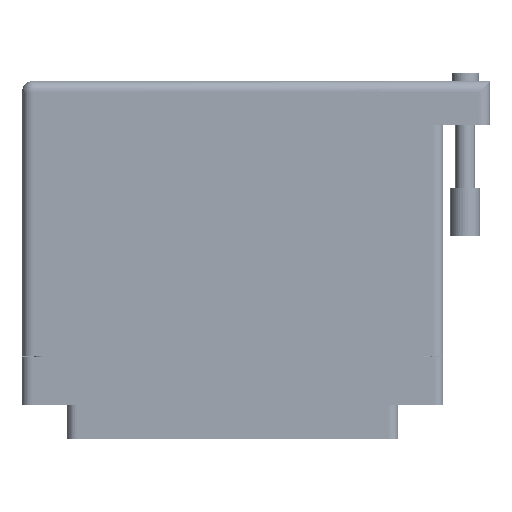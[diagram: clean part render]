
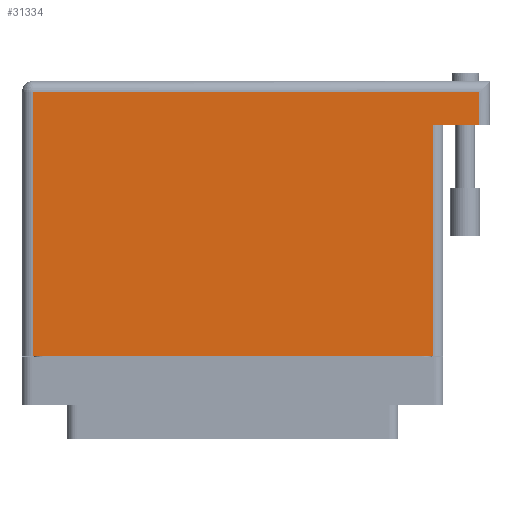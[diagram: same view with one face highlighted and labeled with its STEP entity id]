
A CAD part, front view. The second image highlights one B-rep face of the part: STEP entity #31334.
In plain terms, the highlighted face is planar.
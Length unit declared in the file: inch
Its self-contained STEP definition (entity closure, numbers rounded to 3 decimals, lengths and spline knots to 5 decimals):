
#239 = CARTESIAN_POINT ( 'NONE',  ( -1.289, -0.1, 0.617 ) ) ;
#4967 = ORIENTED_EDGE ( 'NONE', *, *, #35825, .T. ) ;
#5981 = VERTEX_POINT ( 'NONE', #13484 ) ;
#6640 = DIRECTION ( 'NONE',  ( 1., 0., 0. ) ) ;
#6830 = AXIS2_PLACEMENT_3D ( 'NONE', #13305, #51186, #57053 ) ;
#6877 = CARTESIAN_POINT ( 'NONE',  ( -1.359, -0.1, 0.617 ) ) ;
#6927 = ORIENTED_EDGE ( 'NONE', *, *, #57910, .F. ) ;
#8064 = EDGE_CURVE ( 'NONE', #47133, #68225, #53258, .T. ) ;
#10103 = FACE_OUTER_BOUND ( 'NONE', #64344, .T. ) ;
#10275 = ORIENTED_EDGE ( 'NONE', *, *, #18310, .T. ) ;
#11267 = VECTOR ( 'NONE', #66884, 39.37008 ) ;
#12974 = LINE ( 'NONE', #51051, #11267 ) ;
#13305 = CARTESIAN_POINT ( 'NONE',  ( -1.359, 1.675, 0.617 ) ) ;
#13484 = CARTESIAN_POINT ( 'NONE',  ( 1.589, 1.395, 0.617 ) ) ;
#13561 = VECTOR ( 'NONE', #64209, 39.37008 ) ;
#15276 = CARTESIAN_POINT ( 'NONE',  ( 1.289, 1.395, 0.617 ) ) ;
#16328 = ORIENTED_EDGE ( 'NONE', *, *, #60985, .T. ) ;
#17291 = LINE ( 'NONE', #48616, #28340 ) ;
#17690 = LINE ( 'NONE', #68873, #23637 ) ;
#17777 = LINE ( 'NONE', #26431, #13561 ) ;
#18310 = EDGE_CURVE ( 'NONE', #67453, #47133, #17777, .T. ) ;
#22267 = ORIENTED_EDGE ( 'NONE', *, *, #8064, .T. ) ;
#22354 = VECTOR ( 'NONE', #6640, 39.37008 ) ;
#23018 = CARTESIAN_POINT ( 'NONE',  ( -1.289, -0.1, 0.617 ) ) ;
#23637 = VECTOR ( 'NONE', #46229, 39.37008 ) ;
#26431 = CARTESIAN_POINT ( 'NONE',  ( -1.359, 1.605, 0.617 ) ) ;
#27829 = VERTEX_POINT ( 'NONE', #15276 ) ;
#28340 = VECTOR ( 'NONE', #59426, 39.37008 ) ;
#31334 = ADVANCED_FACE ( 'NONE', ( #10103 ), #67724, .F. ) ;
#33004 = ORIENTED_EDGE ( 'NONE', *, *, #51006, .T. ) ;
#34826 = CARTESIAN_POINT ( 'NONE',  ( 1.589, 1.605, 0.617 ) ) ;
#35825 = EDGE_CURVE ( 'NONE', #68225, #41296, #67212, .T. ) ;
#39392 = DIRECTION ( 'NONE',  ( 0., -1., 0. ) ) ;
#41296 = VERTEX_POINT ( 'NONE', #46029 ) ;
#44831 = VECTOR ( 'NONE', #39392, 39.37008 ) ;
#46029 = CARTESIAN_POINT ( 'NONE',  ( 1.289, -0.1, 0.617 ) ) ;
#46229 = DIRECTION ( 'NONE',  ( 0., 1., 0. ) ) ;
#47133 = VERTEX_POINT ( 'NONE', #56104 ) ;
#48616 = CARTESIAN_POINT ( 'NONE',  ( 1.659, 1.395, 0.617 ) ) ;
#51006 = EDGE_CURVE ( 'NONE', #5981, #67453, #17690, .T. ) ;
#51051 = CARTESIAN_POINT ( 'NONE',  ( 1.289, 1.395, 0.617 ) ) ;
#51186 = DIRECTION ( 'NONE',  ( 0., 0., -1. ) ) ;
#53258 = LINE ( 'NONE', #23018, #44831 ) ;
#56104 = CARTESIAN_POINT ( 'NONE',  ( -1.289, 1.605, 0.617 ) ) ;
#57053 = DIRECTION ( 'NONE',  ( -1., 0., 0. ) ) ;
#57910 = EDGE_CURVE ( 'NONE', #5981, #27829, #17291, .T. ) ;
#59426 = DIRECTION ( 'NONE',  ( -1., 0., 0. ) ) ;
#60985 = EDGE_CURVE ( 'NONE', #41296, #27829, #12974, .T. ) ;
#64209 = DIRECTION ( 'NONE',  ( -1., 0., 0. ) ) ;
#64344 = EDGE_LOOP ( 'NONE', ( #4967, #16328, #6927, #33004, #10275, #22267 ) ) ;
#66884 = DIRECTION ( 'NONE',  ( 0., 1., 0. ) ) ;
#67212 = LINE ( 'NONE', #6877, #22354 ) ;
#67453 = VERTEX_POINT ( 'NONE', #34826 ) ;
#67724 = PLANE ( 'NONE',  #6830 ) ;
#68225 = VERTEX_POINT ( 'NONE', #239 ) ;
#68873 = CARTESIAN_POINT ( 'NONE',  ( 1.589, 1.675, 0.617 ) ) ;
